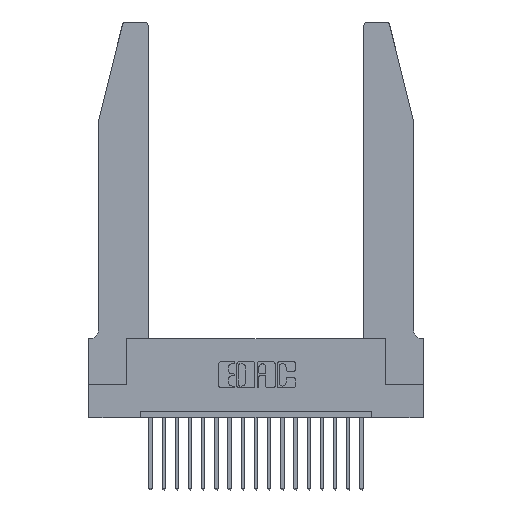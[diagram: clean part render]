
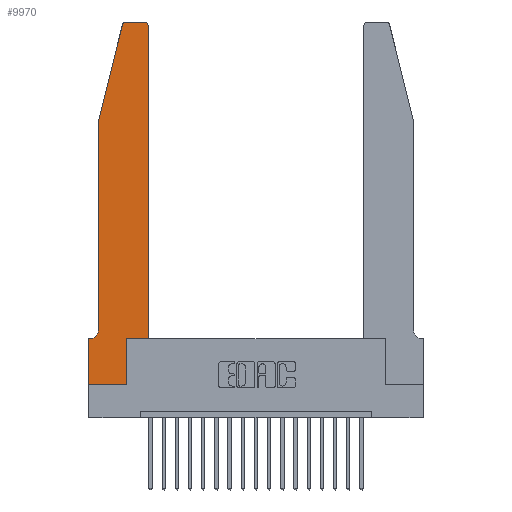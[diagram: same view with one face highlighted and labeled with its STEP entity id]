
A CAD part, top view. The second image highlights one B-rep face of the part: STEP entity #9970.
In plain terms, the highlighted planar face has unit normal (0, 0, 1).
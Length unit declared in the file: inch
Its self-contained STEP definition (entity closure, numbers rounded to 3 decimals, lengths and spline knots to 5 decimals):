
#60 = LINE ( 'NONE', #9650, #15736 ) ;
#205 = CARTESIAN_POINT ( 'NONE',  ( 0.2865, 0.35, 0.37 ) ) ;
#378 = CARTESIAN_POINT ( 'NONE',  ( 0.284, 2.72, 0.37 ) ) ;
#398 = EDGE_CURVE ( 'NONE', #17065, #13692, #12217, .T. ) ;
#671 = CARTESIAN_POINT ( 'NONE',  ( 0.0755, 2., 0.37 ) ) ;
#991 = VECTOR ( 'NONE', #12500, 39.37008 ) ;
#1377 = DIRECTION ( 'NONE',  ( 0., 0., 1. ) ) ;
#1560 = VERTEX_POINT ( 'NONE', #9851 ) ;
#1654 = DIRECTION ( 'NONE',  ( 0., -1., 0. ) ) ;
#2183 = FACE_OUTER_BOUND ( 'NONE', #5867, .T. ) ;
#2679 = LINE ( 'NONE', #8633, #15567 ) ;
#3107 = EDGE_CURVE ( 'NONE', #6061, #16547, #2679, .T. ) ;
#3294 = CARTESIAN_POINT ( 'NONE',  ( 0., 0., 0.37 ) ) ;
#3685 = CIRCLE ( 'NONE', #6583, 0.03 ) ;
#3725 = DIRECTION ( 'NONE',  ( 1., 0., 0. ) ) ;
#4256 = ORIENTED_EDGE ( 'NONE', *, *, #14897, .T. ) ;
#4439 = LINE ( 'NONE', #6014, #4964 ) ;
#4709 = ORIENTED_EDGE ( 'NONE', *, *, #10794, .T. ) ;
#4824 = CARTESIAN_POINT ( 'NONE',  ( 0.4205, 2.72, 0.37 ) ) ;
#4964 = VECTOR ( 'NONE', #12614, 39.37008 ) ;
#4971 = CARTESIAN_POINT ( 'NONE',  ( 0.2865, 0.35, 0.37 ) ) ;
#5061 = EDGE_CURVE ( 'NONE', #18593, #17065, #60, .T. ) ;
#5301 = VECTOR ( 'NONE', #8135, 39.37008 ) ;
#5478 = DIRECTION ( 'NONE',  ( -1., 0., 0. ) ) ;
#5867 = EDGE_LOOP ( 'NONE', ( #4256, #8369, #14037, #15809, #20848, #20382, #20291, #15838, #13515, #13750, #8013, #4709 ) ) ;
#6014 = CARTESIAN_POINT ( 'NONE',  ( 0.0755, 0.35, 0.37 ) ) ;
#6061 = VERTEX_POINT ( 'NONE', #16986 ) ;
#6135 = AXIS2_PLACEMENT_3D ( 'NONE', #378, #16559, #3725 ) ;
#6292 = AXIS2_PLACEMENT_3D ( 'NONE', #13762, #9079, #17163 ) ;
#6323 = CIRCLE ( 'NONE', #6135, 0.03 ) ;
#6583 = AXIS2_PLACEMENT_3D ( 'NONE', #4824, #1377, #11265 ) ;
#6824 = VERTEX_POINT ( 'NONE', #16524 ) ;
#6906 = CARTESIAN_POINT ( 'NONE',  ( 0.0755, 2., 0.37 ) ) ;
#7969 = CARTESIAN_POINT ( 'NONE',  ( 0.25487, 2.72718, 0.37 ) ) ;
#8013 = ORIENTED_EDGE ( 'NONE', *, *, #3107, .T. ) ;
#8054 = CARTESIAN_POINT ( 'NONE',  ( 0.2865, 0., 0.37 ) ) ;
#8135 = DIRECTION ( 'NONE',  ( 0., 1., 0. ) ) ;
#8194 = VERTEX_POINT ( 'NONE', #205 ) ;
#8369 = ORIENTED_EDGE ( 'NONE', *, *, #8455, .T. ) ;
#8419 = DIRECTION ( 'NONE',  ( 0., 1., 0. ) ) ;
#8455 = EDGE_CURVE ( 'NONE', #14833, #10573, #6323, .T. ) ;
#8633 = CARTESIAN_POINT ( 'NONE',  ( 0.4505, 0.35, 0.37 ) ) ;
#8867 = AXIS2_PLACEMENT_3D ( 'NONE', #10133, #16540, #5478 ) ;
#9079 = DIRECTION ( 'NONE',  ( 0., 0., 1. ) ) ;
#9113 = CARTESIAN_POINT ( 'NONE',  ( 0., 0., 0.37 ) ) ;
#9123 = EDGE_CURVE ( 'NONE', #6824, #17544, #16374, .T. ) ;
#9322 = LINE ( 'NONE', #15833, #991 ) ;
#9573 = LINE ( 'NONE', #4971, #5301 ) ;
#9650 = CARTESIAN_POINT ( 'NONE',  ( 0., 0., 0.37 ) ) ;
#9750 = VECTOR ( 'NONE', #15416, 39.37008 ) ;
#9851 = CARTESIAN_POINT ( 'NONE',  ( 0.4205, 2.75, 0.37 ) ) ;
#9970 = ADVANCED_FACE ( 'NONE', ( #2183 ), #12151, .T. ) ;
#10100 = CARTESIAN_POINT ( 'NONE',  ( 0., 0.35, 0.37 ) ) ;
#10133 = CARTESIAN_POINT ( 'NONE',  ( 0.0055, 0.42, 0.37 ) ) ;
#10150 = DIRECTION ( 'NONE',  ( 1., 0., 0. ) ) ;
#10490 = LINE ( 'NONE', #671, #9750 ) ;
#10573 = VERTEX_POINT ( 'NONE', #7969 ) ;
#10652 = EDGE_CURVE ( 'NONE', #10573, #10997, #10490, .T. ) ;
#10794 = EDGE_CURVE ( 'NONE', #16547, #1560, #3685, .T. ) ;
#10997 = VERTEX_POINT ( 'NONE', #6906 ) ;
#11051 = CARTESIAN_POINT ( 'NONE',  ( 0.4505, 0.35, 0.37 ) ) ;
#11265 = DIRECTION ( 'NONE',  ( 1., 0., 0. ) ) ;
#12151 = PLANE ( 'NONE',  #6292 ) ;
#12190 = DIRECTION ( 'NONE',  ( 1., 0., 0. ) ) ;
#12217 = LINE ( 'NONE', #9113, #13480 ) ;
#12500 = DIRECTION ( 'NONE',  ( -1., 0., 0. ) ) ;
#12614 = DIRECTION ( 'NONE',  ( -1., 0., 0. ) ) ;
#12644 = CARTESIAN_POINT ( 'NONE',  ( 0.284, 2.75, 0.37 ) ) ;
#13480 = VECTOR ( 'NONE', #12190, 39.37008 ) ;
#13515 = ORIENTED_EDGE ( 'NONE', *, *, #18394, .T. ) ;
#13594 = CARTESIAN_POINT ( 'NONE',  ( 0.4505, 2.72, 0.37 ) ) ;
#13692 = VERTEX_POINT ( 'NONE', #8054 ) ;
#13750 = ORIENTED_EDGE ( 'NONE', *, *, #16346, .T. ) ;
#13762 = CARTESIAN_POINT ( 'NONE',  ( 0., 0.35, 0.37 ) ) ;
#14023 = LINE ( 'NONE', #19616, #20860 ) ;
#14037 = ORIENTED_EDGE ( 'NONE', *, *, #10652, .T. ) ;
#14833 = VERTEX_POINT ( 'NONE', #12644 ) ;
#14897 = EDGE_CURVE ( 'NONE', #1560, #14833, #9322, .T. ) ;
#15416 = DIRECTION ( 'NONE',  ( -0.239, -0.971, 0. ) ) ;
#15567 = VECTOR ( 'NONE', #8419, 39.37008 ) ;
#15736 = VECTOR ( 'NONE', #1654, 39.37008 ) ;
#15809 = ORIENTED_EDGE ( 'NONE', *, *, #19788, .T. ) ;
#15833 = CARTESIAN_POINT ( 'NONE',  ( 0.2605, 2.75, 0.37 ) ) ;
#15838 = ORIENTED_EDGE ( 'NONE', *, *, #398, .T. ) ;
#16024 = CARTESIAN_POINT ( 'NONE',  ( 0.0055, 0.35, 0.37 ) ) ;
#16346 = EDGE_CURVE ( 'NONE', #8194, #6061, #16698, .T. ) ;
#16374 = CIRCLE ( 'NONE', #8867, 0.07 ) ;
#16524 = CARTESIAN_POINT ( 'NONE',  ( 0.0755, 0.42, 0.37 ) ) ;
#16540 = DIRECTION ( 'NONE',  ( 0., 0., -1. ) ) ;
#16547 = VERTEX_POINT ( 'NONE', #13594 ) ;
#16559 = DIRECTION ( 'NONE',  ( 0., 0., 1. ) ) ;
#16698 = LINE ( 'NONE', #11051, #18437 ) ;
#16986 = CARTESIAN_POINT ( 'NONE',  ( 0.4505, 0.35, 0.37 ) ) ;
#17065 = VERTEX_POINT ( 'NONE', #3294 ) ;
#17163 = DIRECTION ( 'NONE',  ( 1., 0., 0. ) ) ;
#17544 = VERTEX_POINT ( 'NONE', #16024 ) ;
#18394 = EDGE_CURVE ( 'NONE', #13692, #8194, #9573, .T. ) ;
#18437 = VECTOR ( 'NONE', #10150, 39.37008 ) ;
#18593 = VERTEX_POINT ( 'NONE', #10100 ) ;
#19419 = DIRECTION ( 'NONE',  ( 0., -1., 0. ) ) ;
#19616 = CARTESIAN_POINT ( 'NONE',  ( 0.0755, 2., 0.37 ) ) ;
#19788 = EDGE_CURVE ( 'NONE', #10997, #6824, #14023, .T. ) ;
#20186 = EDGE_CURVE ( 'NONE', #17544, #18593, #4439, .T. ) ;
#20291 = ORIENTED_EDGE ( 'NONE', *, *, #5061, .T. ) ;
#20382 = ORIENTED_EDGE ( 'NONE', *, *, #20186, .T. ) ;
#20848 = ORIENTED_EDGE ( 'NONE', *, *, #9123, .T. ) ;
#20860 = VECTOR ( 'NONE', #19419, 39.37008 ) ;
